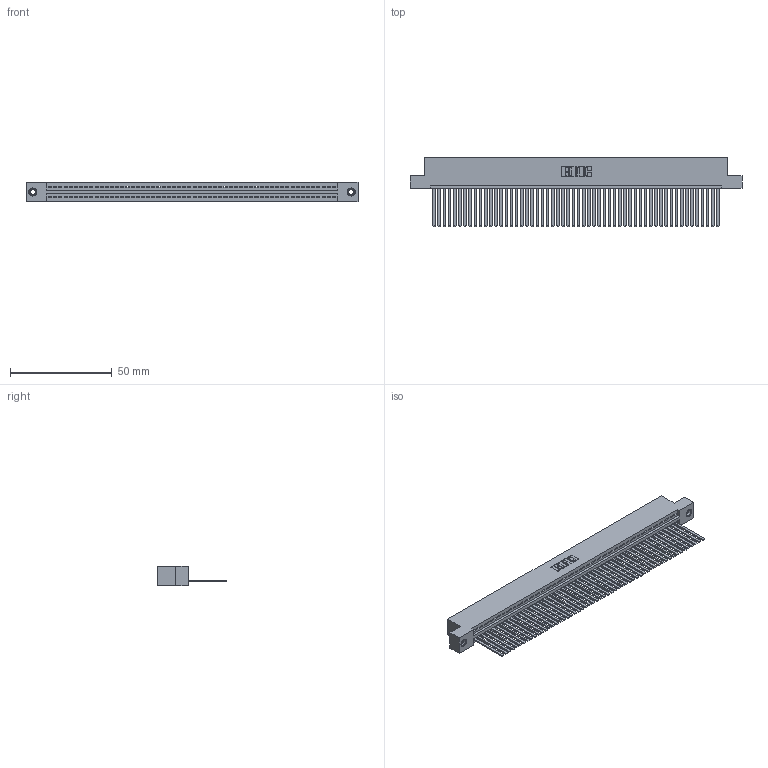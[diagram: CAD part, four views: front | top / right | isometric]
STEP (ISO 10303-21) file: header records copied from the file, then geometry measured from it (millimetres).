
FILE_DESCRIPTION (( 'STEP AP203' ), '1' );
FILE_NAME ('395-056-544-107.STEP', '2019-10-23T23:42:53', ( '' ), ( '' ), 'SwSTEP 2.0', 'SolidWorks 2016', '' );
FILE_SCHEMA (( 'CONFIG_CONTROL_DESIGN' ));
Length unit declared in the file: inch
Products named in the file (4): 395-056-544-107; 345-250-001_345-250-005-103; 345 Part_Flush Mounting Lugs - 0.156 Dia-TI; 345-292-001_345-293-144
Assembly tree (59 placements, depth 2):
  395-056-544-107
    345 Part_Flush Mounting Lugs - 0.156 Dia-TI
    345-292-001_345-293-144  x56
    345-250-001_345-250-005-103  x2
Bounding box: 163.45 x 33.96 x 9.4 mm (x, y, z)
Volume: 16274.3 mm3; surface area: 23796.9 mm2
Topology: 59 solids, 59 shells, 3098 faces, 9325 edges, 6134 vertices
Faces by surface type: plane 2128, cylinder 954, cone 12, torus 4
Entity records: 41264 total; most frequent: CARTESIAN_POINT 7127, ORIENTED_EDGE 7110, DIRECTION 6229, EDGE_CURVE 3555, VECTOR 3183, LINE 3183, VERTEX_POINT 2364, AXIS2_PLACEMENT_3D 1523
